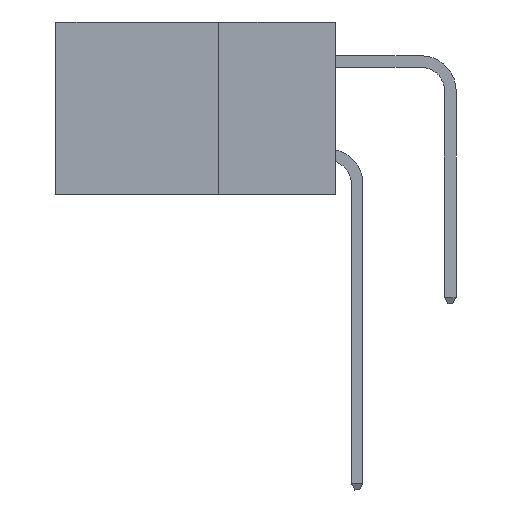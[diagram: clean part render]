
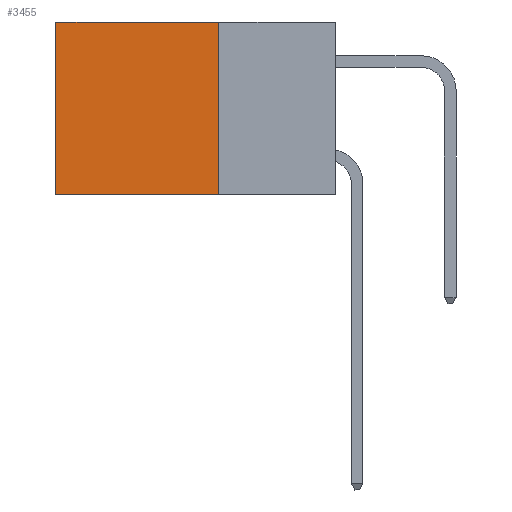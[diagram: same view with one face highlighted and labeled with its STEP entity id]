
A CAD part, left-side view. The second image highlights one B-rep face of the part: STEP entity #3455.
In plain terms, the highlighted planar face has unit normal (-1, 0, 0).
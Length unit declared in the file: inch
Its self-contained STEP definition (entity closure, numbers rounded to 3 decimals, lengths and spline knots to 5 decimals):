
#112 = VERTEX_POINT ( 'NONE', #2187 ) ;
#484 = CARTESIAN_POINT ( 'NONE',  ( 0.2875, 0.25, 0. ) ) ;
#759 = CARTESIAN_POINT ( 'NONE',  ( 0.2875, 0.25, -0.37 ) ) ;
#905 = EDGE_CURVE ( 'NONE', #112, #17516, #21660, .T. ) ;
#1211 = EDGE_CURVE ( 'NONE', #5841, #112, #3211, .T. ) ;
#2166 = DIRECTION ( 'NONE',  ( 0., 1., 0. ) ) ;
#2187 = CARTESIAN_POINT ( 'NONE',  ( 0.2875, 0.6, 0. ) ) ;
#3211 = LINE ( 'NONE', #6473, #22503 ) ;
#3321 = CARTESIAN_POINT ( 'NONE',  ( 0.2875, 0.25, 0. ) ) ;
#3455 = ADVANCED_FACE ( 'NONE', ( #20174 ), #21362, .F. ) ;
#4009 = DIRECTION ( 'NONE',  ( 0., 1., 0. ) ) ;
#4126 = ORIENTED_EDGE ( 'NONE', *, *, #1211, .T. ) ;
#4128 = ORIENTED_EDGE ( 'NONE', *, *, #7874, .F. ) ;
#4924 = CARTESIAN_POINT ( 'NONE',  ( 0.2875, 0.6, -0.37 ) ) ;
#5587 = LINE ( 'NONE', #9260, #12940 ) ;
#5841 = VERTEX_POINT ( 'NONE', #7111 ) ;
#6473 = CARTESIAN_POINT ( 'NONE',  ( 0.2875, 0.25, 0. ) ) ;
#7111 = CARTESIAN_POINT ( 'NONE',  ( 0.2875, 0.25, 0. ) ) ;
#7874 = EDGE_CURVE ( 'NONE', #20499, #17516, #5587, .T. ) ;
#9214 = DIRECTION ( 'NONE',  ( 0., 0., -1. ) ) ;
#9260 = CARTESIAN_POINT ( 'NONE',  ( 0.2875, 0.25, -0.37 ) ) ;
#9733 = ORIENTED_EDGE ( 'NONE', *, *, #905, .T. ) ;
#10790 = DIRECTION ( 'NONE',  ( 1., 0., 0. ) ) ;
#12328 = ORIENTED_EDGE ( 'NONE', *, *, #22065, .F. ) ;
#12940 = VECTOR ( 'NONE', #4009, 39.37008 ) ;
#14549 = DIRECTION ( 'NONE',  ( 0., 0., -1. ) ) ;
#15787 = VECTOR ( 'NONE', #22495, 39.37008 ) ;
#17516 = VERTEX_POINT ( 'NONE', #4924 ) ;
#19012 = AXIS2_PLACEMENT_3D ( 'NONE', #484, #10790, #14549 ) ;
#19369 = LINE ( 'NONE', #3321, #15787 ) ;
#19454 = VECTOR ( 'NONE', #9214, 39.37008 ) ;
#19593 = CARTESIAN_POINT ( 'NONE',  ( 0.2875, 0.6, 0. ) ) ;
#20174 = FACE_OUTER_BOUND ( 'NONE', #22440, .T. ) ;
#20499 = VERTEX_POINT ( 'NONE', #759 ) ;
#21362 = PLANE ( 'NONE',  #19012 ) ;
#21660 = LINE ( 'NONE', #19593, #19454 ) ;
#22065 = EDGE_CURVE ( 'NONE', #5841, #20499, #19369, .T. ) ;
#22440 = EDGE_LOOP ( 'NONE', ( #9733, #4128, #12328, #4126 ) ) ;
#22495 = DIRECTION ( 'NONE',  ( 0., 0., -1. ) ) ;
#22503 = VECTOR ( 'NONE', #2166, 39.37008 ) ;
